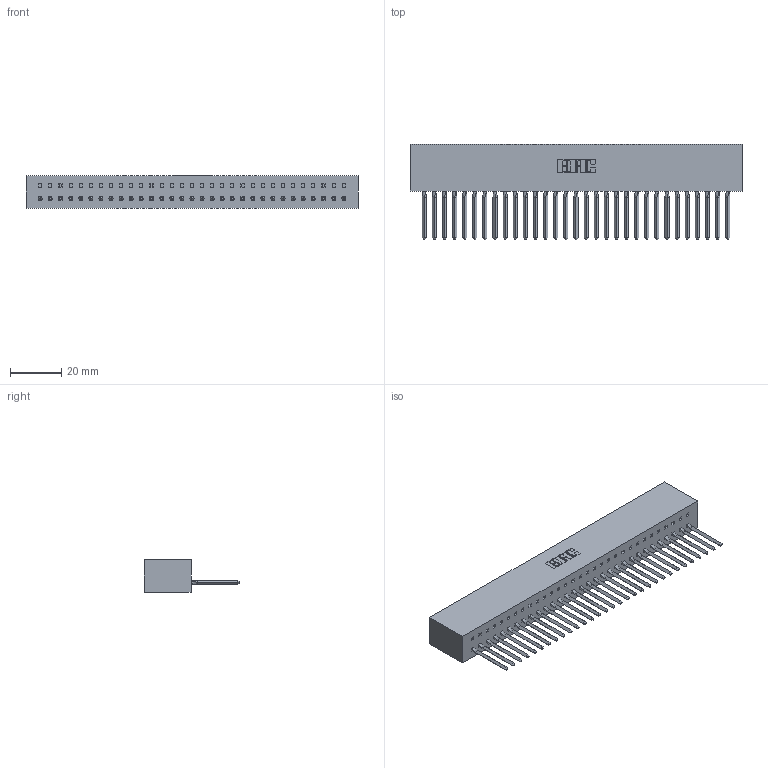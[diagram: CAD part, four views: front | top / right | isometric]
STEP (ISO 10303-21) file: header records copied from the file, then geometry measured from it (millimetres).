
FILE_DESCRIPTION (( 'STEP AP203' ), '1' );
FILE_NAME ('317-031-541-601.STEP', '2020-02-27T20:44:06', ( '' ), ( '' ), 'SwSTEP 2.0', 'SolidWorks 2016', '' );
FILE_SCHEMA (( 'CONFIG_CONTROL_DESIGN' ));
Length unit declared in the file: inch
Products named in the file (3): 317-290-002_541; 317 Part_Lugless; 317-031-541-601
Assembly tree (32 placements, depth 2):
  317-031-541-601
    317 Part_Lugless
    317-290-002_541  x31
Bounding box: 130.05 x 37.34 x 12.7 mm (x, y, z)
Volume: 22457 mm3; surface area: 31560.2 mm2
Topology: 32 solids, 32 shells, 4802 faces, 13693 edges, 8900 vertices
Faces by surface type: plane 3894, cylinder 784, bspline 124
Entity records: 46492 total; most frequent: CARTESIAN_POINT 8902, ORIENTED_EDGE 8186, DIRECTION 6707, EDGE_CURVE 4093, LINE 3737, VECTOR 3737, VERTEX_POINT 2720, AXIS2_PLACEMENT_3D 1485
